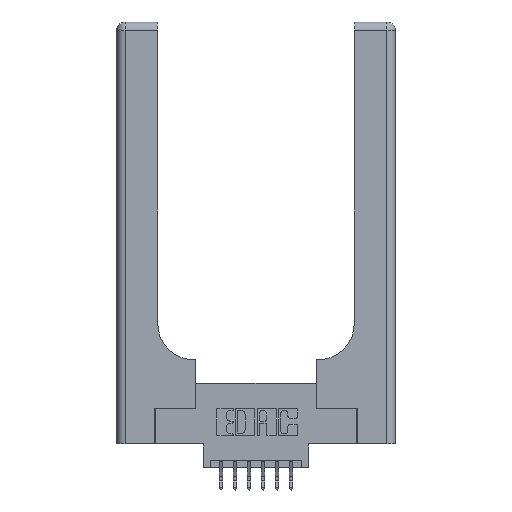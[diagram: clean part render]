
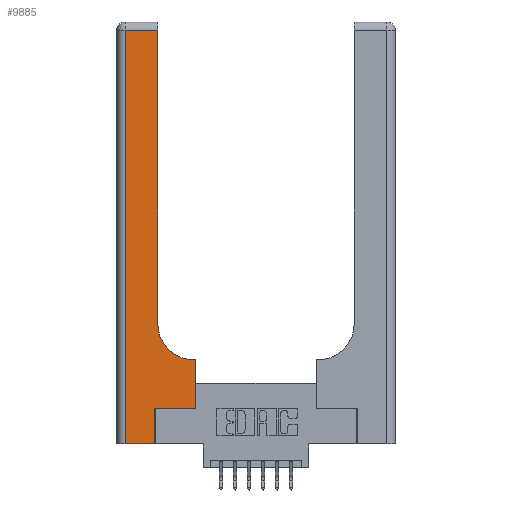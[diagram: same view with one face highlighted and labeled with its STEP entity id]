
A CAD part, top view. The second image highlights one B-rep face of the part: STEP entity #9885.
In plain terms, the highlighted planar face has unit normal (0, 0, 1).
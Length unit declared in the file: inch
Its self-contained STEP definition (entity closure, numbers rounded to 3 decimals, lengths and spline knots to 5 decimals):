
#59 = VECTOR ( 'NONE', #12385, 39.37008 ) ;
#761 = EDGE_CURVE ( 'NONE', #6023, #937, #7909, .T. ) ;
#890 = DIRECTION ( 'NONE',  ( 0., 1., 0. ) ) ;
#937 = VERTEX_POINT ( 'NONE', #4947 ) ;
#1699 = EDGE_CURVE ( 'NONE', #4489, #6023, #12068, .T. ) ;
#1931 = ORIENTED_EDGE ( 'NONE', *, *, #761, .T. ) ;
#2006 = EDGE_CURVE ( 'NONE', #5565, #6816, #14051, .T. ) ;
#2846 = DIRECTION ( 'NONE',  ( -1., 0., 0. ) ) ;
#3014 = ORIENTED_EDGE ( 'NONE', *, *, #8048, .T. ) ;
#3220 = VECTOR ( 'NONE', #7786, 39.37008 ) ;
#3337 = VERTEX_POINT ( 'NONE', #6410 ) ;
#3681 = VECTOR ( 'NONE', #5267, 39.37008 ) ;
#3947 = ORIENTED_EDGE ( 'NONE', *, *, #2006, .T. ) ;
#4069 = CARTESIAN_POINT ( 'NONE',  ( 0.5585, 0.6, 0.37 ) ) ;
#4204 = CARTESIAN_POINT ( 'NONE',  ( 0.269, 0.25, 0.37 ) ) ;
#4403 = CARTESIAN_POINT ( 'NONE',  ( 0.2915, 0.6, 0.37 ) ) ;
#4489 = VERTEX_POINT ( 'NONE', #7762 ) ;
#4537 = AXIS2_PLACEMENT_3D ( 'NONE', #5808, #9439, #8219 ) ;
#4544 = CARTESIAN_POINT ( 'NONE',  ( 0.269, 0.25, 0.37 ) ) ;
#4947 = CARTESIAN_POINT ( 'NONE',  ( 0.06, 0., 0.37 ) ) ;
#5161 = DIRECTION ( 'NONE',  ( 0., 1., 0. ) ) ;
#5267 = DIRECTION ( 'NONE',  ( 0., 1., 0. ) ) ;
#5553 = ORIENTED_EDGE ( 'NONE', *, *, #5777, .T. ) ;
#5565 = VERTEX_POINT ( 'NONE', #7309 ) ;
#5581 = VECTOR ( 'NONE', #5161, 39.37008 ) ;
#5661 = CARTESIAN_POINT ( 'NONE',  ( 0., 0., 0.37 ) ) ;
#5777 = EDGE_CURVE ( 'NONE', #3337, #12816, #9907, .T. ) ;
#5808 = CARTESIAN_POINT ( 'NONE',  ( 0., 3., 0.37 ) ) ;
#6023 = VERTEX_POINT ( 'NONE', #7925 ) ;
#6029 = VECTOR ( 'NONE', #6486, 39.37008 ) ;
#6071 = DIRECTION ( 'NONE',  ( 1., 0., 0. ) ) ;
#6124 = CARTESIAN_POINT ( 'NONE',  ( 0.5415, 0.85, 0.37 ) ) ;
#6410 = CARTESIAN_POINT ( 'NONE',  ( 0.269, 0., 0.37 ) ) ;
#6486 = DIRECTION ( 'NONE',  ( 1., 0., 0. ) ) ;
#6671 = EDGE_CURVE ( 'NONE', #12816, #14416, #10291, .T. ) ;
#6816 = VERTEX_POINT ( 'NONE', #10183 ) ;
#7062 = LINE ( 'NONE', #4403, #3220 ) ;
#7309 = CARTESIAN_POINT ( 'NONE',  ( 0.5415, 0.6, 0.37 ) ) ;
#7371 = CARTESIAN_POINT ( 'NONE',  ( 0.5585, 0.25, 0.37 ) ) ;
#7694 = CARTESIAN_POINT ( 'NONE',  ( 0.06, 3., 0.37 ) ) ;
#7762 = CARTESIAN_POINT ( 'NONE',  ( 0.2915, 2.94, 0.37 ) ) ;
#7786 = DIRECTION ( 'NONE',  ( -1., 0., 0. ) ) ;
#7909 = LINE ( 'NONE', #7694, #59 ) ;
#7925 = CARTESIAN_POINT ( 'NONE',  ( 0.06, 2.94, 0.37 ) ) ;
#7950 = ORIENTED_EDGE ( 'NONE', *, *, #6671, .T. ) ;
#7984 = VECTOR ( 'NONE', #890, 39.37008 ) ;
#8048 = EDGE_CURVE ( 'NONE', #11603, #5565, #7062, .T. ) ;
#8219 = DIRECTION ( 'NONE',  ( -1., 0., 0. ) ) ;
#8392 = EDGE_LOOP ( 'NONE', ( #11737, #15003, #1931, #9853, #5553, #7950, #14156, #3014, #3947 ) ) ;
#8693 = CARTESIAN_POINT ( 'NONE',  ( 0., 2.94, 0.37 ) ) ;
#8702 = LINE ( 'NONE', #12108, #5581 ) ;
#9439 = DIRECTION ( 'NONE',  ( 0., 0., -1. ) ) ;
#9691 = VECTOR ( 'NONE', #2846, 39.37008 ) ;
#9853 = ORIENTED_EDGE ( 'NONE', *, *, #10516, .T. ) ;
#9885 = ADVANCED_FACE ( 'NONE', ( #11441 ), #14077, .F. ) ;
#9907 = LINE ( 'NONE', #10938, #3681 ) ;
#10183 = CARTESIAN_POINT ( 'NONE',  ( 0.2915, 0.85, 0.37 ) ) ;
#10229 = DIRECTION ( 'NONE',  ( 1., 0., 0. ) ) ;
#10291 = LINE ( 'NONE', #4204, #6029 ) ;
#10516 = EDGE_CURVE ( 'NONE', #937, #3337, #13637, .T. ) ;
#10920 = EDGE_CURVE ( 'NONE', #14416, #11603, #8702, .T. ) ;
#10938 = CARTESIAN_POINT ( 'NONE',  ( 0.269, 0., 0.37 ) ) ;
#11095 = AXIS2_PLACEMENT_3D ( 'NONE', #6124, #13069, #6071 ) ;
#11441 = FACE_OUTER_BOUND ( 'NONE', #8392, .T. ) ;
#11603 = VERTEX_POINT ( 'NONE', #4069 ) ;
#11737 = ORIENTED_EDGE ( 'NONE', *, *, #15087, .T. ) ;
#12068 = LINE ( 'NONE', #8693, #9691 ) ;
#12108 = CARTESIAN_POINT ( 'NONE',  ( 0.5585, 0.25, 0.37 ) ) ;
#12362 = LINE ( 'NONE', #14235, #7984 ) ;
#12385 = DIRECTION ( 'NONE',  ( 0., -1., 0. ) ) ;
#12816 = VERTEX_POINT ( 'NONE', #4544 ) ;
#12891 = VECTOR ( 'NONE', #10229, 39.37008 ) ;
#13069 = DIRECTION ( 'NONE',  ( 0., 0., -1. ) ) ;
#13637 = LINE ( 'NONE', #5661, #12891 ) ;
#14051 = CIRCLE ( 'NONE', #11095, 0.25 ) ;
#14077 = PLANE ( 'NONE',  #4537 ) ;
#14156 = ORIENTED_EDGE ( 'NONE', *, *, #10920, .T. ) ;
#14235 = CARTESIAN_POINT ( 'NONE',  ( 0.2915, 3., 0.37 ) ) ;
#14416 = VERTEX_POINT ( 'NONE', #7371 ) ;
#15003 = ORIENTED_EDGE ( 'NONE', *, *, #1699, .T. ) ;
#15087 = EDGE_CURVE ( 'NONE', #6816, #4489, #12362, .T. ) ;
